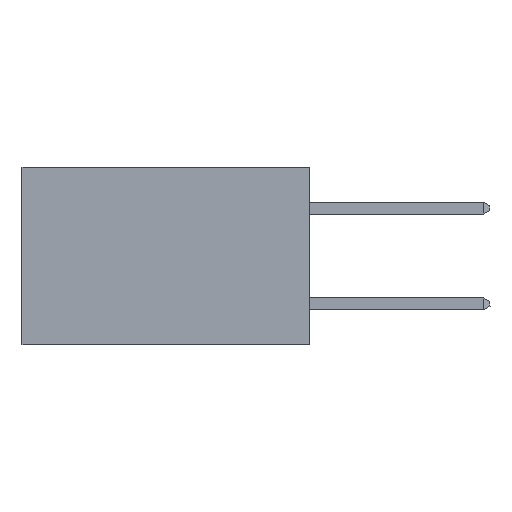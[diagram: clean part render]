
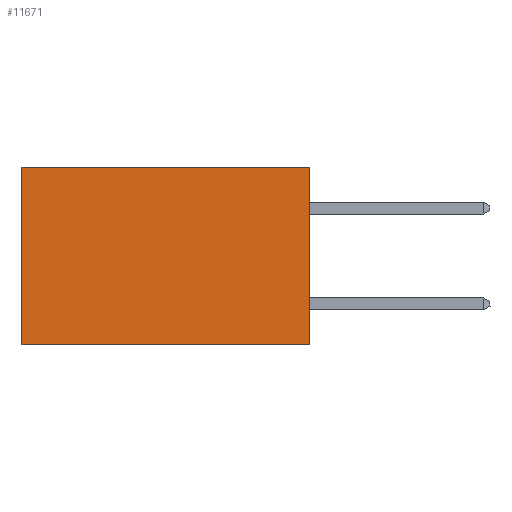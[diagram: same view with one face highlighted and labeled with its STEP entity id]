
A CAD part, left-side view. The second image highlights one B-rep face of the part: STEP entity #11671.
In plain terms, the highlighted planar face has unit normal (-1, 0, 0).
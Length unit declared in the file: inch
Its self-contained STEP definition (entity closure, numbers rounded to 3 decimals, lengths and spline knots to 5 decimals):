
#402 = VECTOR ( 'NONE', #5828, 39.37008 ) ;
#501 = PLANE ( 'NONE',  #9326 ) ;
#708 = EDGE_CURVE ( 'NONE', #5741, #11952, #2021, .T. ) ;
#836 = EDGE_CURVE ( 'NONE', #11952, #10918, #2663, .T. ) ;
#1521 = VECTOR ( 'NONE', #2091, 39.37008 ) ;
#1872 = DIRECTION ( 'NONE',  ( 0., 0., -1. ) ) ;
#1956 = VERTEX_POINT ( 'NONE', #9959 ) ;
#2021 = LINE ( 'NONE', #16094, #15351 ) ;
#2091 = DIRECTION ( 'NONE',  ( 0., 0., -1. ) ) ;
#2663 = LINE ( 'NONE', #9939, #9974 ) ;
#3103 = CARTESIAN_POINT ( 'NONE',  ( 0.2875, 0., -0.37 ) ) ;
#5327 = LINE ( 'NONE', #3103, #402 ) ;
#5741 = VERTEX_POINT ( 'NONE', #15945 ) ;
#5786 = ORIENTED_EDGE ( 'NONE', *, *, #10503, .F. ) ;
#5828 = DIRECTION ( 'NONE',  ( 0., 1., 0. ) ) ;
#6991 = CARTESIAN_POINT ( 'NONE',  ( 0.2875, 0.6, -0.37 ) ) ;
#9050 = ORIENTED_EDGE ( 'NONE', *, *, #836, .T. ) ;
#9124 = EDGE_CURVE ( 'NONE', #1956, #10918, #5327, .T. ) ;
#9326 = AXIS2_PLACEMENT_3D ( 'NONE', #11455, #10114, #1872 ) ;
#9939 = CARTESIAN_POINT ( 'NONE',  ( 0.2875, 0.6, 0. ) ) ;
#9959 = CARTESIAN_POINT ( 'NONE',  ( 0.2875, 0., -0.37 ) ) ;
#9974 = VECTOR ( 'NONE', #11213, 39.37008 ) ;
#10114 = DIRECTION ( 'NONE',  ( 1., 0., 0. ) ) ;
#10340 = CARTESIAN_POINT ( 'NONE',  ( 0.2875, 0., 0. ) ) ;
#10503 = EDGE_CURVE ( 'NONE', #5741, #1956, #12082, .T. ) ;
#10918 = VERTEX_POINT ( 'NONE', #6991 ) ;
#11213 = DIRECTION ( 'NONE',  ( 0., 0., -1. ) ) ;
#11455 = CARTESIAN_POINT ( 'NONE',  ( 0.2875, 0., 0. ) ) ;
#11671 = ADVANCED_FACE ( 'NONE', ( #17343 ), #501, .F. ) ;
#11952 = VERTEX_POINT ( 'NONE', #14745 ) ;
#12082 = LINE ( 'NONE', #10340, #1521 ) ;
#12785 = EDGE_LOOP ( 'NONE', ( #9050, #16345, #5786, #16761 ) ) ;
#14745 = CARTESIAN_POINT ( 'NONE',  ( 0.2875, 0.6, 0. ) ) ;
#15351 = VECTOR ( 'NONE', #15933, 39.37008 ) ;
#15933 = DIRECTION ( 'NONE',  ( 0., 1., 0. ) ) ;
#15945 = CARTESIAN_POINT ( 'NONE',  ( 0.2875, 0., 0. ) ) ;
#16094 = CARTESIAN_POINT ( 'NONE',  ( 0.2875, 0., 0. ) ) ;
#16345 = ORIENTED_EDGE ( 'NONE', *, *, #9124, .F. ) ;
#16761 = ORIENTED_EDGE ( 'NONE', *, *, #708, .T. ) ;
#17343 = FACE_OUTER_BOUND ( 'NONE', #12785, .T. ) ;
